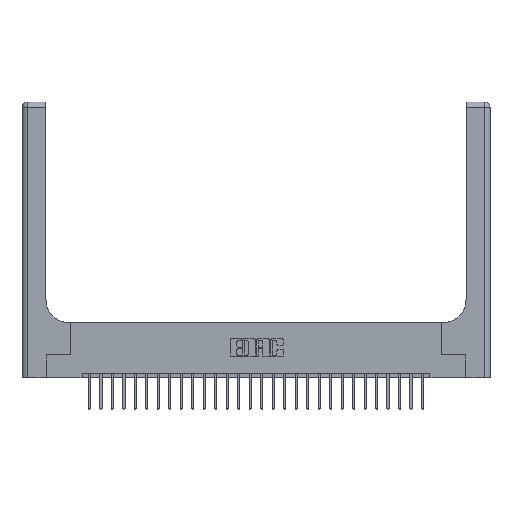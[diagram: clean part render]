
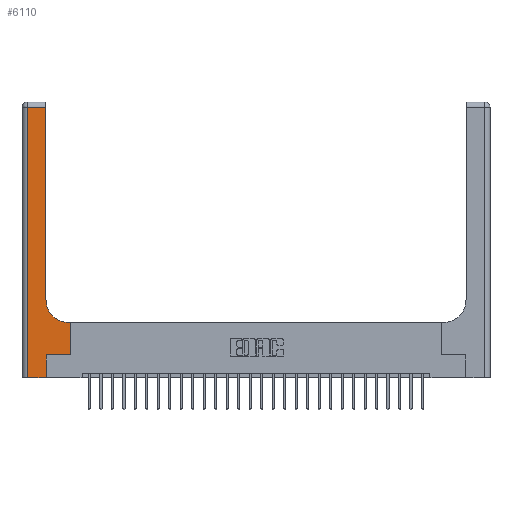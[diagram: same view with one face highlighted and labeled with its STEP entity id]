
A CAD part, top view. The second image highlights one B-rep face of the part: STEP entity #6110.
In plain terms, the highlighted planar face has unit normal (0, 0, 1).
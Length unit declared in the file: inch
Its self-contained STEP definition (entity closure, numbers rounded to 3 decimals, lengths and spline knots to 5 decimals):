
#50 = EDGE_CURVE ( 'NONE', #11118, #16682, #3244, .T. ) ;
#718 = EDGE_CURVE ( 'NONE', #23059, #14041, #5131, .T. ) ;
#1344 = CARTESIAN_POINT ( 'NONE',  ( 0.26, 2.94, 0.37 ) ) ;
#1550 = ORIENTED_EDGE ( 'NONE', *, *, #11135, .T. ) ;
#2002 = CARTESIAN_POINT ( 'NONE',  ( 0.26, 0.85, 0.37 ) ) ;
#2188 = CARTESIAN_POINT ( 'NONE',  ( 0.265, 0.25, 0.37 ) ) ;
#2403 = EDGE_CURVE ( 'NONE', #16564, #11898, #8876, .T. ) ;
#2406 = VERTEX_POINT ( 'NONE', #6701 ) ;
#2744 = CARTESIAN_POINT ( 'NONE',  ( 0.528, 0.25, 0.37 ) ) ;
#2922 = LINE ( 'NONE', #24813, #12521 ) ;
#3044 = ORIENTED_EDGE ( 'NONE', *, *, #11262, .T. ) ;
#3120 = DIRECTION ( 'NONE',  ( -1., 0., 0. ) ) ;
#3159 = VERTEX_POINT ( 'NONE', #2188 ) ;
#3244 = LINE ( 'NONE', #5067, #4173 ) ;
#4173 = VECTOR ( 'NONE', #20633, 39.37008 ) ;
#4315 = FACE_OUTER_BOUND ( 'NONE', #8733, .T. ) ;
#4704 = DIRECTION ( 'NONE',  ( 0., 1., 0. ) ) ;
#5067 = CARTESIAN_POINT ( 'NONE',  ( 0.06, 3., 0.37 ) ) ;
#5126 = CARTESIAN_POINT ( 'NONE',  ( 0.528, 0.25, 0.37 ) ) ;
#5131 = CIRCLE ( 'NONE', #21463, 0.25 ) ;
#5309 = CARTESIAN_POINT ( 'NONE',  ( 0., 0., 0.37 ) ) ;
#5382 = CARTESIAN_POINT ( 'NONE',  ( 0.51, 0.85, 0.37 ) ) ;
#6110 = ADVANCED_FACE ( 'NONE', ( #4315 ), #8793, .F. ) ;
#6690 = CARTESIAN_POINT ( 'NONE',  ( 0.51, 0.6, 0.37 ) ) ;
#6701 = CARTESIAN_POINT ( 'NONE',  ( 0.265, 0., 0.37 ) ) ;
#6808 = CARTESIAN_POINT ( 'NONE',  ( 0.528, 0.6, 0.37 ) ) ;
#7898 = ORIENTED_EDGE ( 'NONE', *, *, #2403, .T. ) ;
#8528 = ORIENTED_EDGE ( 'NONE', *, *, #718, .T. ) ;
#8733 = EDGE_LOOP ( 'NONE', ( #1550, #22872, #10364, #17261, #3044, #23155, #7898, #17747, #8528 ) ) ;
#8793 = PLANE ( 'NONE',  #16439 ) ;
#8876 = LINE ( 'NONE', #2744, #11715 ) ;
#9471 = DIRECTION ( 'NONE',  ( 1., 0., 0. ) ) ;
#10364 = ORIENTED_EDGE ( 'NONE', *, *, #50, .T. ) ;
#10854 = EDGE_CURVE ( 'NONE', #11898, #23059, #23069, .T. ) ;
#11118 = VERTEX_POINT ( 'NONE', #24500 ) ;
#11135 = EDGE_CURVE ( 'NONE', #14041, #20225, #21155, .T. ) ;
#11262 = EDGE_CURVE ( 'NONE', #2406, #3159, #15105, .T. ) ;
#11532 = DIRECTION ( 'NONE',  ( 1., 0., 0. ) ) ;
#11715 = VECTOR ( 'NONE', #25233, 39.37008 ) ;
#11756 = EDGE_CURVE ( 'NONE', #20225, #11118, #2922, .T. ) ;
#11898 = VERTEX_POINT ( 'NONE', #6808 ) ;
#12353 = EDGE_CURVE ( 'NONE', #3159, #16564, #20770, .T. ) ;
#12521 = VECTOR ( 'NONE', #18935, 39.37008 ) ;
#14041 = VERTEX_POINT ( 'NONE', #2002 ) ;
#14708 = VECTOR ( 'NONE', #21384, 39.37008 ) ;
#15105 = LINE ( 'NONE', #17020, #17642 ) ;
#15404 = VECTOR ( 'NONE', #16219, 39.37008 ) ;
#16219 = DIRECTION ( 'NONE',  ( 0., 1., 0. ) ) ;
#16246 = CARTESIAN_POINT ( 'NONE',  ( 0.06, 0., 0.37 ) ) ;
#16439 = AXIS2_PLACEMENT_3D ( 'NONE', #18844, #25089, #21072 ) ;
#16564 = VERTEX_POINT ( 'NONE', #5126 ) ;
#16682 = VERTEX_POINT ( 'NONE', #16246 ) ;
#17020 = CARTESIAN_POINT ( 'NONE',  ( 0.265, 0., 0.37 ) ) ;
#17223 = CARTESIAN_POINT ( 'NONE',  ( 0.26, 0.6, 0.37 ) ) ;
#17261 = ORIENTED_EDGE ( 'NONE', *, *, #25584, .T. ) ;
#17642 = VECTOR ( 'NONE', #4704, 39.37008 ) ;
#17747 = ORIENTED_EDGE ( 'NONE', *, *, #10854, .T. ) ;
#18844 = CARTESIAN_POINT ( 'NONE',  ( 0., 3., 0.37 ) ) ;
#18935 = DIRECTION ( 'NONE',  ( -1., 0., 0. ) ) ;
#20063 = CARTESIAN_POINT ( 'NONE',  ( 0.26, 3., 0.37 ) ) ;
#20225 = VERTEX_POINT ( 'NONE', #1344 ) ;
#20633 = DIRECTION ( 'NONE',  ( 0., -1., 0. ) ) ;
#20770 = LINE ( 'NONE', #22524, #14708 ) ;
#21072 = DIRECTION ( 'NONE',  ( -1., 0., 0. ) ) ;
#21155 = LINE ( 'NONE', #20063, #15404 ) ;
#21384 = DIRECTION ( 'NONE',  ( 1., 0., 0. ) ) ;
#21463 = AXIS2_PLACEMENT_3D ( 'NONE', #5382, #25780, #9471 ) ;
#21727 = VECTOR ( 'NONE', #11532, 39.37008 ) ;
#22378 = LINE ( 'NONE', #5309, #21727 ) ;
#22524 = CARTESIAN_POINT ( 'NONE',  ( 0.265, 0.25, 0.37 ) ) ;
#22872 = ORIENTED_EDGE ( 'NONE', *, *, #11756, .T. ) ;
#23059 = VERTEX_POINT ( 'NONE', #6690 ) ;
#23069 = LINE ( 'NONE', #17223, #25638 ) ;
#23155 = ORIENTED_EDGE ( 'NONE', *, *, #12353, .T. ) ;
#24500 = CARTESIAN_POINT ( 'NONE',  ( 0.06, 2.94, 0.37 ) ) ;
#24813 = CARTESIAN_POINT ( 'NONE',  ( 0., 2.94, 0.37 ) ) ;
#25089 = DIRECTION ( 'NONE',  ( 0., 0., -1. ) ) ;
#25233 = DIRECTION ( 'NONE',  ( 0., 1., 0. ) ) ;
#25584 = EDGE_CURVE ( 'NONE', #16682, #2406, #22378, .T. ) ;
#25638 = VECTOR ( 'NONE', #3120, 39.37008 ) ;
#25780 = DIRECTION ( 'NONE',  ( 0., 0., -1. ) ) ;
